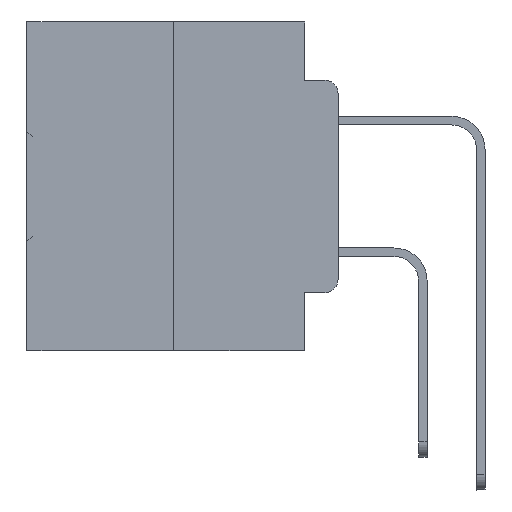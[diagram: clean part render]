
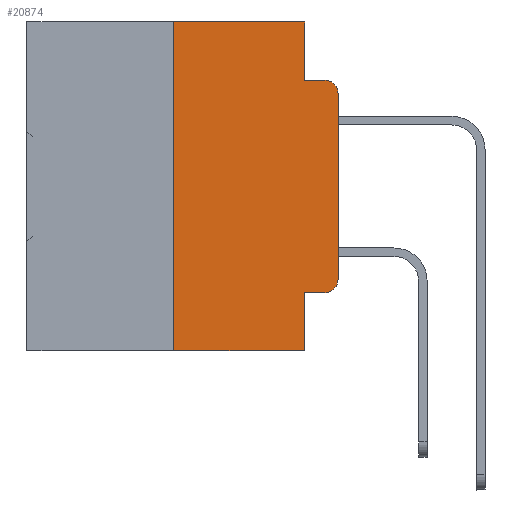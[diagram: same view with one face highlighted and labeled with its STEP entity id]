
A CAD part, left-side view. The second image highlights one B-rep face of the part: STEP entity #20874.
In plain terms, the highlighted planar face has unit normal (-1, 0, 0).
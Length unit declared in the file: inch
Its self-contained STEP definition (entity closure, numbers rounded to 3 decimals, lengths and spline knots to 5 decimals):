
#117 = DIRECTION ( 'NONE',  ( -1., 0., 0. ) ) ;
#204 = DIRECTION ( 'NONE',  ( 0., 0., -1. ) ) ;
#1416 = VECTOR ( 'NONE', #20642, 39.37008 ) ;
#1695 = CARTESIAN_POINT ( 'NONE',  ( 0., 0.051, 0. ) ) ;
#2225 = ORIENTED_EDGE ( 'NONE', *, *, #19444, .F. ) ;
#2868 = EDGE_CURVE ( 'NONE', #31850, #17282, #24808, .T. ) ;
#3663 = ORIENTED_EDGE ( 'NONE', *, *, #29701, .T. ) ;
#4974 = VECTOR ( 'NONE', #17539, 39.37008 ) ;
#7588 = EDGE_CURVE ( 'NONE', #15505, #13856, #13068, .T. ) ;
#7637 = EDGE_LOOP ( 'NONE', ( #22024, #16095, #2225, #18881, #20687, #35827, #8745, #18438, #3663, #27829 ) ) ;
#7881 = VERTEX_POINT ( 'NONE', #20838 ) ;
#8745 = ORIENTED_EDGE ( 'NONE', *, *, #30671, .T. ) ;
#9351 = AXIS2_PLACEMENT_3D ( 'NONE', #17895, #117, #20803 ) ;
#9529 = FACE_OUTER_BOUND ( 'NONE', #7637, .T. ) ;
#9565 = EDGE_CURVE ( 'NONE', #14807, #25230, #19623, .T. ) ;
#10480 = LINE ( 'NONE', #19525, #17407 ) ;
#10912 = VERTEX_POINT ( 'NONE', #18891 ) ;
#10948 = CIRCLE ( 'NONE', #9351, 0.02 ) ;
#11086 = LINE ( 'NONE', #28763, #26539 ) ;
#11396 = DIRECTION ( 'NONE',  ( 0., -1., 0. ) ) ;
#11679 = CARTESIAN_POINT ( 'NONE',  ( 0., 0.25, 0. ) ) ;
#11728 = VECTOR ( 'NONE', #30202, 39.37008 ) ;
#11796 = AXIS2_PLACEMENT_3D ( 'NONE', #35079, #17978, #204 ) ;
#11998 = PLANE ( 'NONE',  #11796 ) ;
#12137 = VECTOR ( 'NONE', #13823, 39.37008 ) ;
#12789 = LINE ( 'NONE', #14572, #4974 ) ;
#13068 = LINE ( 'NONE', #36783, #12137 ) ;
#13434 = CARTESIAN_POINT ( 'NONE',  ( 0., 0., 0. ) ) ;
#13823 = DIRECTION ( 'NONE',  ( 0., 0., 1. ) ) ;
#13856 = VERTEX_POINT ( 'NONE', #11679 ) ;
#14572 = CARTESIAN_POINT ( 'NONE',  ( 0., 0.051, -0.0885 ) ) ;
#14807 = VERTEX_POINT ( 'NONE', #1695 ) ;
#15072 = DIRECTION ( 'NONE',  ( 0., -1., 0. ) ) ;
#15483 = VECTOR ( 'NONE', #35411, 39.37008 ) ;
#15505 = VERTEX_POINT ( 'NONE', #35165 ) ;
#16095 = ORIENTED_EDGE ( 'NONE', *, *, #21354, .T. ) ;
#16257 = DIRECTION ( 'NONE',  ( -1., 0., 0. ) ) ;
#17282 = VERTEX_POINT ( 'NONE', #26693 ) ;
#17407 = VECTOR ( 'NONE', #30855, 39.37008 ) ;
#17539 = DIRECTION ( 'NONE',  ( 0., -1., 0. ) ) ;
#17895 = CARTESIAN_POINT ( 'NONE',  ( 0., 0.02, -0.3915 ) ) ;
#17978 = DIRECTION ( 'NONE',  ( 1., 0., 0. ) ) ;
#18258 = VERTEX_POINT ( 'NONE', #26135 ) ;
#18438 = ORIENTED_EDGE ( 'NONE', *, *, #31610, .F. ) ;
#18881 = ORIENTED_EDGE ( 'NONE', *, *, #9565, .F. ) ;
#18891 = CARTESIAN_POINT ( 'NONE',  ( 0., 0.02, -0.4115 ) ) ;
#19444 = EDGE_CURVE ( 'NONE', #25230, #33331, #12789, .T. ) ;
#19525 = CARTESIAN_POINT ( 'NONE',  ( 0., 0.473, -0.5 ) ) ;
#19623 = LINE ( 'NONE', #24480, #11728 ) ;
#20153 = EDGE_CURVE ( 'NONE', #10912, #31850, #10948, .T. ) ;
#20642 = DIRECTION ( 'NONE',  ( 0., 0., 1. ) ) ;
#20687 = ORIENTED_EDGE ( 'NONE', *, *, #37341, .F. ) ;
#20803 = DIRECTION ( 'NONE',  ( 0., 0., -1. ) ) ;
#20838 = CARTESIAN_POINT ( 'NONE',  ( 0., 0.051, -0.4115 ) ) ;
#20874 = ADVANCED_FACE ( 'NONE', ( #9529 ), #11998, .F. ) ;
#21196 = CARTESIAN_POINT ( 'NONE',  ( 0., 0.02, -0.0885 ) ) ;
#21354 = EDGE_CURVE ( 'NONE', #17282, #33331, #35137, .T. ) ;
#22024 = ORIENTED_EDGE ( 'NONE', *, *, #2868, .T. ) ;
#23709 = CARTESIAN_POINT ( 'NONE',  ( 0., 0.051, -0.4115 ) ) ;
#24391 = CARTESIAN_POINT ( 'NONE',  ( 0., 0.051, -0.0885 ) ) ;
#24480 = CARTESIAN_POINT ( 'NONE',  ( 0., 0.051, 0. ) ) ;
#24808 = LINE ( 'NONE', #13434, #1416 ) ;
#25230 = VERTEX_POINT ( 'NONE', #24391 ) ;
#26135 = CARTESIAN_POINT ( 'NONE',  ( 0., 0.051, -0.5 ) ) ;
#26539 = VECTOR ( 'NONE', #11396, 39.37008 ) ;
#26693 = CARTESIAN_POINT ( 'NONE',  ( 0., 0., -0.1085 ) ) ;
#27812 = VECTOR ( 'NONE', #15072, 39.37008 ) ;
#27829 = ORIENTED_EDGE ( 'NONE', *, *, #20153, .T. ) ;
#28763 = CARTESIAN_POINT ( 'NONE',  ( 0., 0.473, 0. ) ) ;
#29701 = EDGE_CURVE ( 'NONE', #7881, #10912, #35382, .T. ) ;
#30202 = DIRECTION ( 'NONE',  ( 0., 0., -1. ) ) ;
#30671 = EDGE_CURVE ( 'NONE', #15505, #18258, #10480, .T. ) ;
#30855 = DIRECTION ( 'NONE',  ( 0., -1., 0. ) ) ;
#31610 = EDGE_CURVE ( 'NONE', #7881, #18258, #32569, .T. ) ;
#31850 = VERTEX_POINT ( 'NONE', #33437 ) ;
#32554 = CARTESIAN_POINT ( 'NONE',  ( 0., 0.051, 0. ) ) ;
#32569 = LINE ( 'NONE', #32554, #15483 ) ;
#32900 = AXIS2_PLACEMENT_3D ( 'NONE', #33457, #16257, #36286 ) ;
#33331 = VERTEX_POINT ( 'NONE', #21196 ) ;
#33437 = CARTESIAN_POINT ( 'NONE',  ( 0., 0., -0.3915 ) ) ;
#33457 = CARTESIAN_POINT ( 'NONE',  ( 0., 0.02, -0.1085 ) ) ;
#35079 = CARTESIAN_POINT ( 'NONE',  ( 0., 0.473, 0. ) ) ;
#35137 = CIRCLE ( 'NONE', #32900, 0.02 ) ;
#35165 = CARTESIAN_POINT ( 'NONE',  ( 0., 0.25, -0.5 ) ) ;
#35382 = LINE ( 'NONE', #23709, #27812 ) ;
#35411 = DIRECTION ( 'NONE',  ( 0., 0., -1. ) ) ;
#35827 = ORIENTED_EDGE ( 'NONE', *, *, #7588, .F. ) ;
#36286 = DIRECTION ( 'NONE',  ( 0., 0., -1. ) ) ;
#36783 = CARTESIAN_POINT ( 'NONE',  ( 0., 0.25, 0. ) ) ;
#37341 = EDGE_CURVE ( 'NONE', #13856, #14807, #11086, .T. ) ;
